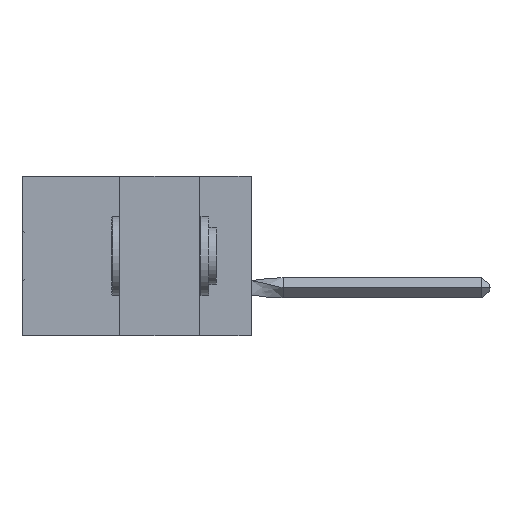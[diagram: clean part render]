
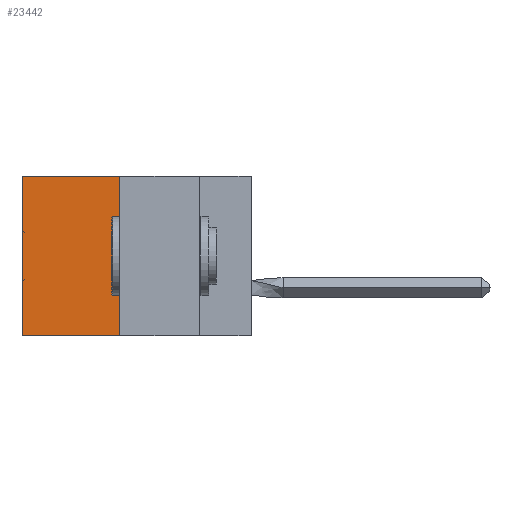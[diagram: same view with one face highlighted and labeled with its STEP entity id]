
A CAD part, left-side view. The second image highlights one B-rep face of the part: STEP entity #23442.
In plain terms, the highlighted planar face has unit normal (-1, 0, 0).
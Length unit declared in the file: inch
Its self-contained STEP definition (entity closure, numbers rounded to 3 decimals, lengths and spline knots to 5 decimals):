
#1526 = EDGE_LOOP ( 'NONE', ( #43217, #15038, #18353, #53588 ) ) ;
#4892 = AXIS2_PLACEMENT_3D ( 'NONE', #26191, #18363, #43289 ) ;
#5633 = VERTEX_POINT ( 'NONE', #44229 ) ;
#7139 = CARTESIAN_POINT ( 'NONE',  ( 0.305, 0.413, 0. ) ) ;
#7316 = DIRECTION ( 'NONE',  ( 0., 1., 0. ) ) ;
#10351 = CARTESIAN_POINT ( 'NONE',  ( 0.305, 0.413, -0.5 ) ) ;
#11152 = EDGE_CURVE ( 'NONE', #50359, #25028, #50958, .T. ) ;
#11671 = VECTOR ( 'NONE', #15572, 39.37008 ) ;
#15038 = ORIENTED_EDGE ( 'NONE', *, *, #47195, .F. ) ;
#15572 = DIRECTION ( 'NONE',  ( 0., 0., -1. ) ) ;
#18353 = ORIENTED_EDGE ( 'NONE', *, *, #26057, .F. ) ;
#18363 = DIRECTION ( 'NONE',  ( 1., 0., 0. ) ) ;
#19173 = EDGE_CURVE ( 'NONE', #32318, #50359, #40508, .T. ) ;
#23442 = ADVANCED_FACE ( 'NONE', ( #48350 ), #26403, .F. ) ;
#25028 = VERTEX_POINT ( 'NONE', #36966 ) ;
#26057 = EDGE_CURVE ( 'NONE', #32318, #5633, #40772, .T. ) ;
#26191 = CARTESIAN_POINT ( 'NONE',  ( 0.305, 0.413, -0.5 ) ) ;
#26403 = PLANE ( 'NONE',  #4892 ) ;
#32318 = VERTEX_POINT ( 'NONE', #46091 ) ;
#35160 = LINE ( 'NONE', #35253, #51289 ) ;
#35253 = CARTESIAN_POINT ( 'NONE',  ( 0.305, 0.413, -0.5 ) ) ;
#36966 = CARTESIAN_POINT ( 'NONE',  ( 0.305, 0.72, -0.5 ) ) ;
#40002 = DIRECTION ( 'NONE',  ( 0., 1., 0. ) ) ;
#40056 = DIRECTION ( 'NONE',  ( 0., 0., -1. ) ) ;
#40508 = LINE ( 'NONE', #7139, #54561 ) ;
#40772 = LINE ( 'NONE', #10351, #50765 ) ;
#43217 = ORIENTED_EDGE ( 'NONE', *, *, #11152, .T. ) ;
#43289 = DIRECTION ( 'NONE',  ( 0., 0., -1. ) ) ;
#44229 = CARTESIAN_POINT ( 'NONE',  ( 0.305, 0.413, -0.5 ) ) ;
#46091 = CARTESIAN_POINT ( 'NONE',  ( 0.305, 0.413, 0. ) ) ;
#47195 = EDGE_CURVE ( 'NONE', #5633, #25028, #35160, .T. ) ;
#48350 = FACE_OUTER_BOUND ( 'NONE', #1526, .T. ) ;
#50342 = CARTESIAN_POINT ( 'NONE',  ( 0.305, 0.72, 0. ) ) ;
#50359 = VERTEX_POINT ( 'NONE', #50342 ) ;
#50765 = VECTOR ( 'NONE', #40056, 39.37008 ) ;
#50958 = LINE ( 'NONE', #53795, #11671 ) ;
#51289 = VECTOR ( 'NONE', #40002, 39.37008 ) ;
#53588 = ORIENTED_EDGE ( 'NONE', *, *, #19173, .T. ) ;
#53795 = CARTESIAN_POINT ( 'NONE',  ( 0.305, 0.72, -0.5 ) ) ;
#54561 = VECTOR ( 'NONE', #7316, 39.37008 ) ;
